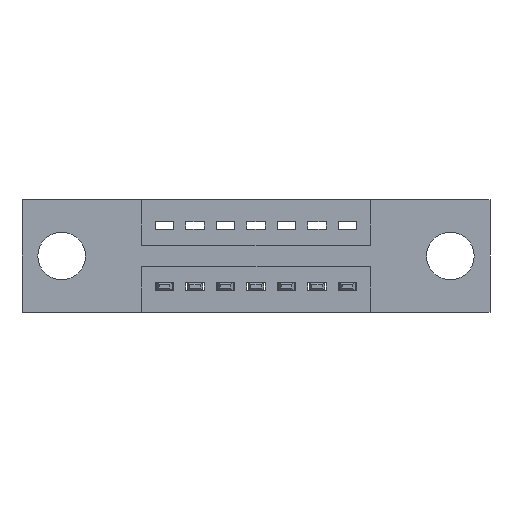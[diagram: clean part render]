
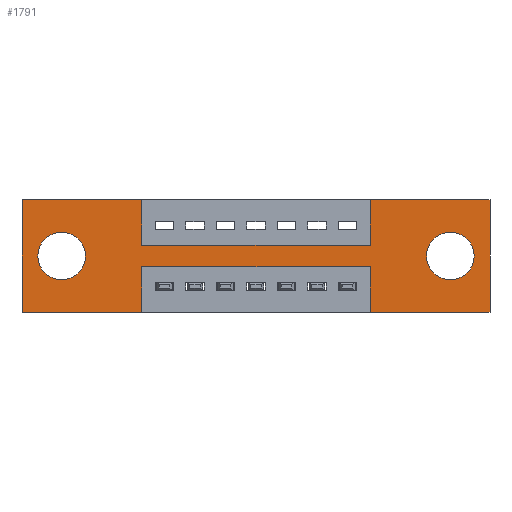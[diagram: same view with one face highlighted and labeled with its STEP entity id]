
A CAD part, front view. The second image highlights one B-rep face of the part: STEP entity #1791.
In plain terms, the highlighted planar face has unit normal (0, -1, 0).
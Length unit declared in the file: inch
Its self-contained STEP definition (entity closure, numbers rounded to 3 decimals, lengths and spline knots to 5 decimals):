
#36 = VERTEX_POINT ( 'NONE', #4985 ) ;
#76 = DIRECTION ( 'NONE',  ( 1., 0., 0. ) ) ;
#108 = LINE ( 'NONE', #2731, #2456 ) ;
#197 = DIRECTION ( 'NONE',  ( 0., 0., -1. ) ) ;
#230 = VERTEX_POINT ( 'NONE', #4171 ) ;
#393 = DIRECTION ( 'NONE',  ( 1., 0., 0. ) ) ;
#516 = EDGE_LOOP ( 'NONE', ( #2111, #1101 ) ) ;
#634 = CARTESIAN_POINT ( 'NONE',  ( 1.1425, 0., 0. ) ) ;
#655 = CARTESIAN_POINT ( 'NONE',  ( 1.405, 0., -0.263 ) ) ;
#693 = ORIENTED_EDGE ( 'NONE', *, *, #5717, .F. ) ;
#704 = EDGE_LOOP ( 'NONE', ( #693, #1035, #8669, #5693, #2913, #3175, #3404, #5851, #8319, #4718, #3060, #1761 ) ) ;
#811 = DIRECTION ( 'NONE',  ( 0., 0., 1. ) ) ;
#966 = VERTEX_POINT ( 'NONE', #634 ) ;
#1035 = ORIENTED_EDGE ( 'NONE', *, *, #8338, .F. ) ;
#1082 = EDGE_CURVE ( 'NONE', #966, #1644, #9069, .T. ) ;
#1101 = ORIENTED_EDGE ( 'NONE', *, *, #1256, .T. ) ;
#1122 = VERTEX_POINT ( 'NONE', #2272 ) ;
#1223 = CARTESIAN_POINT ( 'NONE',  ( 0.13, 0., -0.107 ) ) ;
#1256 = EDGE_CURVE ( 'NONE', #1122, #1851, #5753, .T. ) ;
#1268 = LINE ( 'NONE', #8665, #8967 ) ;
#1269 = LINE ( 'NONE', #5500, #7321 ) ;
#1428 = VECTOR ( 'NONE', #7513, 39.37008 ) ;
#1506 = AXIS2_PLACEMENT_3D ( 'NONE', #6028, #4192, #811 ) ;
#1512 = EDGE_CURVE ( 'NONE', #1851, #1122, #9343, .T. ) ;
#1563 = VERTEX_POINT ( 'NONE', #655 ) ;
#1644 = VERTEX_POINT ( 'NONE', #6504 ) ;
#1751 = EDGE_CURVE ( 'NONE', #5655, #1927, #108, .T. ) ;
#1761 = ORIENTED_EDGE ( 'NONE', *, *, #1751, .F. ) ;
#1771 = EDGE_CURVE ( 'NONE', #5385, #966, #2188, .T. ) ;
#1784 = LINE ( 'NONE', #2864, #8435 ) ;
#1791 = ADVANCED_FACE ( 'NONE', ( #7888, #9335, #4206 ), #2634, .T. ) ;
#1816 = CARTESIAN_POINT ( 'NONE',  ( 0.3925, 0., 0. ) ) ;
#1851 = VERTEX_POINT ( 'NONE', #1223 ) ;
#1902 = LINE ( 'NONE', #6045, #9361 ) ;
#1927 = VERTEX_POINT ( 'NONE', #3520 ) ;
#2111 = ORIENTED_EDGE ( 'NONE', *, *, #1512, .T. ) ;
#2153 = CARTESIAN_POINT ( 'NONE',  ( 1.405, 0., -0.107 ) ) ;
#2187 = CARTESIAN_POINT ( 'NONE',  ( 0.3925, 0., -0.15 ) ) ;
#2188 = LINE ( 'NONE', #8483, #4478 ) ;
#2263 = CARTESIAN_POINT ( 'NONE',  ( 0.3925, 0., -0.22 ) ) ;
#2272 = CARTESIAN_POINT ( 'NONE',  ( 0.13, 0., -0.263 ) ) ;
#2319 = EDGE_CURVE ( 'NONE', #1927, #3568, #5829, .T. ) ;
#2456 = VECTOR ( 'NONE', #7387, 39.37008 ) ;
#2634 = PLANE ( 'NONE',  #6521 ) ;
#2731 = CARTESIAN_POINT ( 'NONE',  ( 0., 0., -0.37 ) ) ;
#2864 = CARTESIAN_POINT ( 'NONE',  ( 1.535, 0., 0. ) ) ;
#2913 = ORIENTED_EDGE ( 'NONE', *, *, #4818, .F. ) ;
#2925 = ORIENTED_EDGE ( 'NONE', *, *, #7859, .T. ) ;
#2931 = VECTOR ( 'NONE', #393, 39.37008 ) ;
#2996 = VERTEX_POINT ( 'NONE', #2263 ) ;
#3052 = DIRECTION ( 'NONE',  ( 0., 1., 0. ) ) ;
#3060 = ORIENTED_EDGE ( 'NONE', *, *, #2319, .F. ) ;
#3123 = VERTEX_POINT ( 'NONE', #2153 ) ;
#3175 = ORIENTED_EDGE ( 'NONE', *, *, #1082, .F. ) ;
#3203 = DIRECTION ( 'NONE',  ( 0., 1., 0. ) ) ;
#3400 = LINE ( 'NONE', #1816, #6893 ) ;
#3404 = ORIENTED_EDGE ( 'NONE', *, *, #1771, .F. ) ;
#3455 = AXIS2_PLACEMENT_3D ( 'NONE', #7973, #6752, #6473 ) ;
#3498 = LINE ( 'NONE', #3797, #2931 ) ;
#3520 = CARTESIAN_POINT ( 'NONE',  ( 0., 0., -0.37 ) ) ;
#3564 = CARTESIAN_POINT ( 'NONE',  ( 1.1425, 0., -0.15 ) ) ;
#3568 = VERTEX_POINT ( 'NONE', #7123 ) ;
#3755 = EDGE_CURVE ( 'NONE', #230, #7154, #3400, .T. ) ;
#3797 = CARTESIAN_POINT ( 'NONE',  ( 0., 0., 0. ) ) ;
#3817 = DIRECTION ( 'NONE',  ( -1., 0., 0. ) ) ;
#3831 = VERTEX_POINT ( 'NONE', #5974 ) ;
#3991 = DIRECTION ( 'NONE',  ( 0., -1., 0. ) ) ;
#4171 = CARTESIAN_POINT ( 'NONE',  ( 0.3925, 0., 0. ) ) ;
#4192 = DIRECTION ( 'NONE',  ( 0., 1., 0. ) ) ;
#4206 = FACE_OUTER_BOUND ( 'NONE', #704, .T. ) ;
#4288 = EDGE_LOOP ( 'NONE', ( #8660, #2925 ) ) ;
#4304 = AXIS2_PLACEMENT_3D ( 'NONE', #7546, #3203, #8173 ) ;
#4478 = VECTOR ( 'NONE', #7506, 39.37008 ) ;
#4479 = CARTESIAN_POINT ( 'NONE',  ( 0., 0., 0. ) ) ;
#4514 = CIRCLE ( 'NONE', #6080, 0.078 ) ;
#4718 = ORIENTED_EDGE ( 'NONE', *, *, #5682, .F. ) ;
#4818 = EDGE_CURVE ( 'NONE', #1644, #3831, #1784, .T. ) ;
#4887 = VECTOR ( 'NONE', #8647, 39.37008 ) ;
#4985 = CARTESIAN_POINT ( 'NONE',  ( 1.1425, 0., -0.22 ) ) ;
#5347 = VERTEX_POINT ( 'NONE', #9630 ) ;
#5385 = VERTEX_POINT ( 'NONE', #3564 ) ;
#5500 = CARTESIAN_POINT ( 'NONE',  ( 1.1425, 0., -0.37 ) ) ;
#5655 = VERTEX_POINT ( 'NONE', #6737 ) ;
#5658 = VECTOR ( 'NONE', #7285, 39.37008 ) ;
#5682 = EDGE_CURVE ( 'NONE', #3568, #230, #3498, .T. ) ;
#5693 = ORIENTED_EDGE ( 'NONE', *, *, #6546, .F. ) ;
#5717 = EDGE_CURVE ( 'NONE', #2996, #5655, #6753, .T. ) ;
#5753 = CIRCLE ( 'NONE', #3455, 0.078 ) ;
#5780 = DIRECTION ( 'NONE',  ( 0., 0., 1. ) ) ;
#5829 = LINE ( 'NONE', #6515, #7587 ) ;
#5851 = ORIENTED_EDGE ( 'NONE', *, *, #6616, .F. ) ;
#5974 = CARTESIAN_POINT ( 'NONE',  ( 1.535, 0., -0.37 ) ) ;
#6028 = CARTESIAN_POINT ( 'NONE',  ( 0.13, 0., -0.185 ) ) ;
#6045 = CARTESIAN_POINT ( 'NONE',  ( 0., 0., -0.37 ) ) ;
#6080 = AXIS2_PLACEMENT_3D ( 'NONE', #7435, #3052, #8068 ) ;
#6104 = CIRCLE ( 'NONE', #4304, 0.078 ) ;
#6197 = DIRECTION ( 'NONE',  ( 0., 0., 1. ) ) ;
#6473 = DIRECTION ( 'NONE',  ( 0., 0., 1. ) ) ;
#6504 = CARTESIAN_POINT ( 'NONE',  ( 1.535, 0., 0. ) ) ;
#6515 = CARTESIAN_POINT ( 'NONE',  ( 0., 0., 0. ) ) ;
#6521 = AXIS2_PLACEMENT_3D ( 'NONE', #7052, #3991, #197 ) ;
#6546 = EDGE_CURVE ( 'NONE', #3831, #5347, #1902, .T. ) ;
#6616 = EDGE_CURVE ( 'NONE', #7154, #5385, #1268, .T. ) ;
#6658 = CARTESIAN_POINT ( 'NONE',  ( 0.3925, 0., -0.22 ) ) ;
#6737 = CARTESIAN_POINT ( 'NONE',  ( 0.3925, 0., -0.37 ) ) ;
#6752 = DIRECTION ( 'NONE',  ( 0., 1., 0. ) ) ;
#6753 = LINE ( 'NONE', #7381, #4887 ) ;
#6893 = VECTOR ( 'NONE', #7873, 39.37008 ) ;
#7052 = CARTESIAN_POINT ( 'NONE',  ( 0., 0., -0.37 ) ) ;
#7123 = CARTESIAN_POINT ( 'NONE',  ( 0., 0., 0. ) ) ;
#7154 = VERTEX_POINT ( 'NONE', #2187 ) ;
#7285 = DIRECTION ( 'NONE',  ( -1., 0., 0. ) ) ;
#7321 = VECTOR ( 'NONE', #6197, 39.37008 ) ;
#7381 = CARTESIAN_POINT ( 'NONE',  ( 0.3925, 0., -0.37 ) ) ;
#7387 = DIRECTION ( 'NONE',  ( -1., 0., 0. ) ) ;
#7435 = CARTESIAN_POINT ( 'NONE',  ( 1.405, 0., -0.185 ) ) ;
#7506 = DIRECTION ( 'NONE',  ( 0., 0., 1. ) ) ;
#7513 = DIRECTION ( 'NONE',  ( 1., 0., 0. ) ) ;
#7546 = CARTESIAN_POINT ( 'NONE',  ( 1.405, 0., -0.185 ) ) ;
#7587 = VECTOR ( 'NONE', #5780, 39.37008 ) ;
#7859 = EDGE_CURVE ( 'NONE', #1563, #3123, #6104, .T. ) ;
#7873 = DIRECTION ( 'NONE',  ( 0., 0., -1. ) ) ;
#7888 = FACE_BOUND ( 'NONE', #4288, .T. ) ;
#7973 = CARTESIAN_POINT ( 'NONE',  ( 0.13, 0., -0.185 ) ) ;
#8068 = DIRECTION ( 'NONE',  ( 0., 0., -1. ) ) ;
#8173 = DIRECTION ( 'NONE',  ( 0., 0., -1. ) ) ;
#8319 = ORIENTED_EDGE ( 'NONE', *, *, #3755, .F. ) ;
#8338 = EDGE_CURVE ( 'NONE', #36, #2996, #9087, .T. ) ;
#8435 = VECTOR ( 'NONE', #8584, 39.37008 ) ;
#8483 = CARTESIAN_POINT ( 'NONE',  ( 1.1425, 0., 0. ) ) ;
#8584 = DIRECTION ( 'NONE',  ( 0., 0., -1. ) ) ;
#8647 = DIRECTION ( 'NONE',  ( 0., 0., -1. ) ) ;
#8660 = ORIENTED_EDGE ( 'NONE', *, *, #9319, .T. ) ;
#8665 = CARTESIAN_POINT ( 'NONE',  ( 0.3925, 0., -0.15 ) ) ;
#8669 = ORIENTED_EDGE ( 'NONE', *, *, #9427, .F. ) ;
#8967 = VECTOR ( 'NONE', #76, 39.37008 ) ;
#9069 = LINE ( 'NONE', #4479, #1428 ) ;
#9087 = LINE ( 'NONE', #6658, #5658 ) ;
#9319 = EDGE_CURVE ( 'NONE', #3123, #1563, #4514, .T. ) ;
#9335 = FACE_BOUND ( 'NONE', #516, .T. ) ;
#9343 = CIRCLE ( 'NONE', #1506, 0.078 ) ;
#9361 = VECTOR ( 'NONE', #3817, 39.37008 ) ;
#9427 = EDGE_CURVE ( 'NONE', #5347, #36, #1269, .T. ) ;
#9630 = CARTESIAN_POINT ( 'NONE',  ( 1.1425, 0., -0.37 ) ) ;
